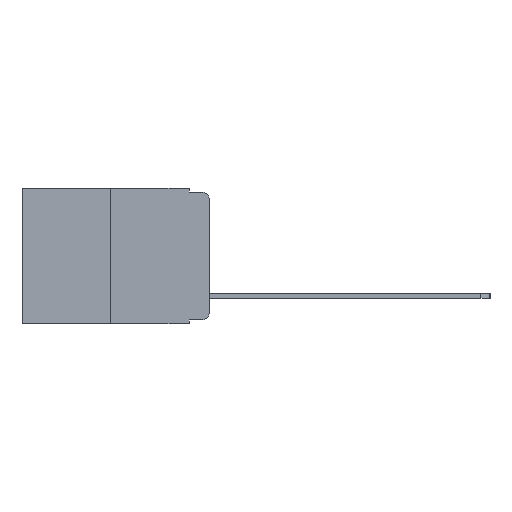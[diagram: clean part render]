
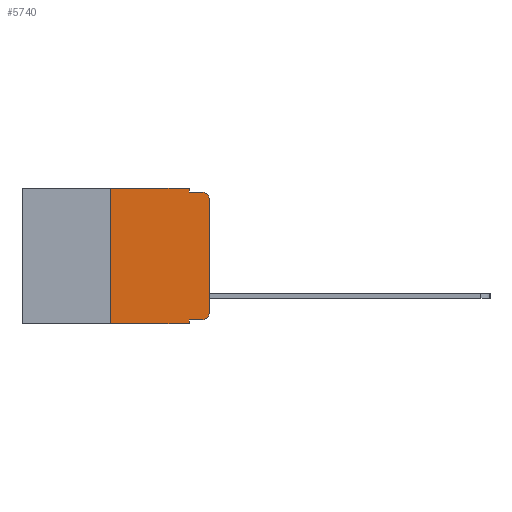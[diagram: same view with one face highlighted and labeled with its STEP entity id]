
A CAD part, left-side view. The second image highlights one B-rep face of the part: STEP entity #5740.
In plain terms, the highlighted planar face has unit normal (-1, 0, 0).
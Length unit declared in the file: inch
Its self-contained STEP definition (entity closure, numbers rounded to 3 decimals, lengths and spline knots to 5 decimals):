
#294 = DIRECTION ( 'NONE',  ( -1., 0., 0. ) ) ;
#671 = CARTESIAN_POINT ( 'NONE',  ( 0., 0., 0. ) ) ;
#924 = CARTESIAN_POINT ( 'NONE',  ( 0., 0.25, 0. ) ) ;
#1082 = CARTESIAN_POINT ( 'NONE',  ( 0., 0.051, -0.343 ) ) ;
#1091 = LINE ( 'NONE', #14338, #14787 ) ;
#1209 = VERTEX_POINT ( 'NONE', #1242 ) ;
#1242 = CARTESIAN_POINT ( 'NONE',  ( 0., 0.02, -0.333 ) ) ;
#1355 = VECTOR ( 'NONE', #15765, 39.37008 ) ;
#1677 = VERTEX_POINT ( 'NONE', #1082 ) ;
#1719 = VECTOR ( 'NONE', #15276, 39.37008 ) ;
#1775 = DIRECTION ( 'NONE',  ( 0., -1., 0. ) ) ;
#1788 = DIRECTION ( 'NONE',  ( 0., 0., -1. ) ) ;
#2135 = EDGE_CURVE ( 'NONE', #14291, #1677, #15732, .T. ) ;
#2163 = VECTOR ( 'NONE', #1775, 39.37008 ) ;
#2519 = CARTESIAN_POINT ( 'NONE',  ( 0., 0.051, -0.01 ) ) ;
#2876 = VERTEX_POINT ( 'NONE', #12834 ) ;
#3567 = CARTESIAN_POINT ( 'NONE',  ( 0., 0.051, -0.333 ) ) ;
#4300 = VERTEX_POINT ( 'NONE', #924 ) ;
#4766 = CARTESIAN_POINT ( 'NONE',  ( 0., 0.051, 0. ) ) ;
#4980 = DIRECTION ( 'NONE',  ( 0., -1., 0. ) ) ;
#5591 = AXIS2_PLACEMENT_3D ( 'NONE', #8691, #294, #9993 ) ;
#5740 = ADVANCED_FACE ( 'NONE', ( #8794 ), #13743, .F. ) ;
#5831 = VECTOR ( 'NONE', #10466, 39.37008 ) ;
#5834 = CARTESIAN_POINT ( 'NONE',  ( 0., 0.02, -0.03 ) ) ;
#5901 = EDGE_CURVE ( 'NONE', #7542, #4300, #13146, .T. ) ;
#6305 = EDGE_CURVE ( 'NONE', #4300, #17138, #15220, .T. ) ;
#6391 = DIRECTION ( 'NONE',  ( 0., 0., 1. ) ) ;
#6464 = EDGE_CURVE ( 'NONE', #17138, #7415, #8756, .T. ) ;
#6732 = VECTOR ( 'NONE', #6391, 39.37008 ) ;
#6981 = ORIENTED_EDGE ( 'NONE', *, *, #16457, .T. ) ;
#7187 = ORIENTED_EDGE ( 'NONE', *, *, #9204, .T. ) ;
#7241 = DIRECTION ( 'NONE',  ( 0., 0., -1. ) ) ;
#7305 = ORIENTED_EDGE ( 'NONE', *, *, #2135, .F. ) ;
#7397 = EDGE_CURVE ( 'NONE', #7415, #8403, #1091, .T. ) ;
#7415 = VERTEX_POINT ( 'NONE', #2519 ) ;
#7450 = CARTESIAN_POINT ( 'NONE',  ( 0., 0.02, -0.01 ) ) ;
#7467 = ORIENTED_EDGE ( 'NONE', *, *, #6305, .F. ) ;
#7485 = ORIENTED_EDGE ( 'NONE', *, *, #12552, .T. ) ;
#7542 = VERTEX_POINT ( 'NONE', #17070 ) ;
#7590 = CARTESIAN_POINT ( 'NONE',  ( 0., 0.473, 0. ) ) ;
#7830 = ORIENTED_EDGE ( 'NONE', *, *, #14002, .T. ) ;
#8237 = ORIENTED_EDGE ( 'NONE', *, *, #11397, .T. ) ;
#8278 = CARTESIAN_POINT ( 'NONE',  ( 0., 0.051, 0. ) ) ;
#8403 = VERTEX_POINT ( 'NONE', #7450 ) ;
#8484 = ORIENTED_EDGE ( 'NONE', *, *, #5901, .F. ) ;
#8535 = ORIENTED_EDGE ( 'NONE', *, *, #6464, .F. ) ;
#8565 = VECTOR ( 'NONE', #9127, 39.37008 ) ;
#8573 = CIRCLE ( 'NONE', #14033, 0.02 ) ;
#8691 = CARTESIAN_POINT ( 'NONE',  ( 0., 0.02, -0.313 ) ) ;
#8756 = LINE ( 'NONE', #8278, #1355 ) ;
#8794 = FACE_OUTER_BOUND ( 'NONE', #12404, .T. ) ;
#8834 = ORIENTED_EDGE ( 'NONE', *, *, #7397, .F. ) ;
#9127 = DIRECTION ( 'NONE',  ( 0., -1., 0. ) ) ;
#9204 = EDGE_CURVE ( 'NONE', #7542, #1677, #9461, .T. ) ;
#9337 = CIRCLE ( 'NONE', #5591, 0.02 ) ;
#9363 = DIRECTION ( 'NONE',  ( 0., -1., 0. ) ) ;
#9461 = LINE ( 'NONE', #10012, #2163 ) ;
#9993 = DIRECTION ( 'NONE',  ( 0., 0., -1. ) ) ;
#10012 = CARTESIAN_POINT ( 'NONE',  ( 0., 0.473, -0.343 ) ) ;
#10024 = DIRECTION ( 'NONE',  ( 1., 0., 0. ) ) ;
#10228 = LINE ( 'NONE', #671, #6732 ) ;
#10363 = CARTESIAN_POINT ( 'NONE',  ( 0., 0.051, 0. ) ) ;
#10466 = DIRECTION ( 'NONE',  ( 0., 0., 1. ) ) ;
#10489 = CARTESIAN_POINT ( 'NONE',  ( 0., 0.051, -0.333 ) ) ;
#10833 = VECTOR ( 'NONE', #4980, 39.37008 ) ;
#11397 = EDGE_CURVE ( 'NONE', #2876, #16993, #10228, .T. ) ;
#11996 = AXIS2_PLACEMENT_3D ( 'NONE', #14954, #10024, #1788 ) ;
#12404 = EDGE_LOOP ( 'NONE', ( #8237, #7485, #8834, #8535, #7467, #8484, #7187, #7305, #6981, #7830 ) ) ;
#12552 = EDGE_CURVE ( 'NONE', #16993, #8403, #8573, .T. ) ;
#12834 = CARTESIAN_POINT ( 'NONE',  ( 0., 0., -0.313 ) ) ;
#13146 = LINE ( 'NONE', #15374, #5831 ) ;
#13743 = PLANE ( 'NONE',  #11996 ) ;
#14002 = EDGE_CURVE ( 'NONE', #1209, #2876, #9337, .T. ) ;
#14033 = AXIS2_PLACEMENT_3D ( 'NONE', #5834, #14796, #7241 ) ;
#14137 = LINE ( 'NONE', #3567, #10833 ) ;
#14291 = VERTEX_POINT ( 'NONE', #10489 ) ;
#14338 = CARTESIAN_POINT ( 'NONE',  ( 0., 0.051, -0.01 ) ) ;
#14787 = VECTOR ( 'NONE', #9363, 39.37008 ) ;
#14796 = DIRECTION ( 'NONE',  ( -1., 0., 0. ) ) ;
#14954 = CARTESIAN_POINT ( 'NONE',  ( 0., 0.473, 0. ) ) ;
#15220 = LINE ( 'NONE', #7590, #8565 ) ;
#15276 = DIRECTION ( 'NONE',  ( 0., 0., -1. ) ) ;
#15374 = CARTESIAN_POINT ( 'NONE',  ( 0., 0.25, 0. ) ) ;
#15732 = LINE ( 'NONE', #4766, #1719 ) ;
#15765 = DIRECTION ( 'NONE',  ( 0., 0., -1. ) ) ;
#16301 = CARTESIAN_POINT ( 'NONE',  ( 0., 0., -0.03 ) ) ;
#16457 = EDGE_CURVE ( 'NONE', #14291, #1209, #14137, .T. ) ;
#16993 = VERTEX_POINT ( 'NONE', #16301 ) ;
#17070 = CARTESIAN_POINT ( 'NONE',  ( 0., 0.25, -0.343 ) ) ;
#17138 = VERTEX_POINT ( 'NONE', #10363 ) ;
